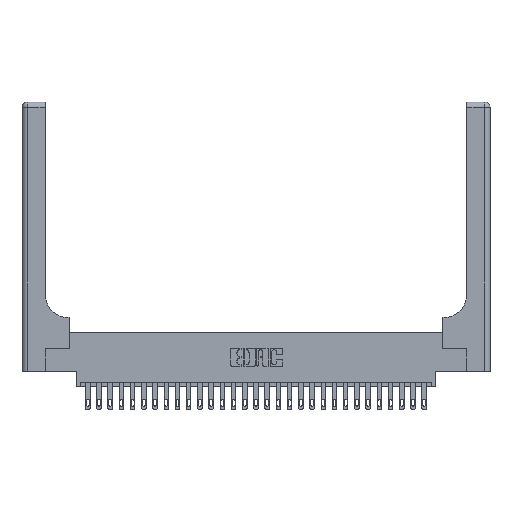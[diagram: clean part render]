
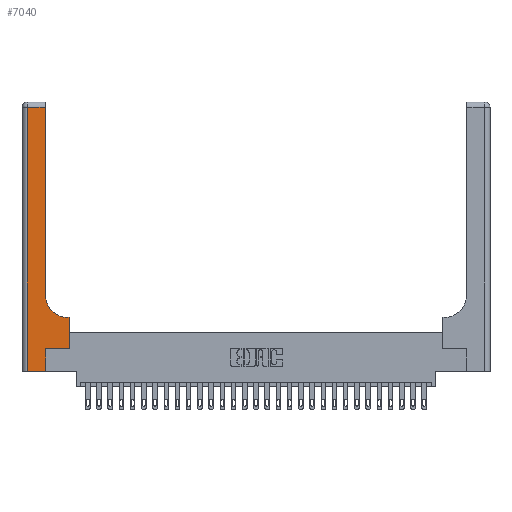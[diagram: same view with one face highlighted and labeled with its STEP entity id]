
A CAD part, top view. The second image highlights one B-rep face of the part: STEP entity #7040.
In plain terms, the highlighted planar face has unit normal (0, 0, 1).
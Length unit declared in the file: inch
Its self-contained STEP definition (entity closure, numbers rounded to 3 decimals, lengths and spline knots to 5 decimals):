
#105 = VERTEX_POINT ( 'NONE', #22768 ) ;
#300 = CARTESIAN_POINT ( 'NONE',  ( 0.528, 0.25, 0.37 ) ) ;
#528 = CARTESIAN_POINT ( 'NONE',  ( 0.265, 0., 0.37 ) ) ;
#1163 = EDGE_CURVE ( 'NONE', #9780, #12907, #8367, .T. ) ;
#1201 = ORIENTED_EDGE ( 'NONE', *, *, #1163, .T. ) ;
#1216 = DIRECTION ( 'NONE',  ( 1., 0., 0. ) ) ;
#1411 = LINE ( 'NONE', #24992, #21447 ) ;
#1665 = DIRECTION ( 'NONE',  ( 0., 0., -1. ) ) ;
#1756 = CARTESIAN_POINT ( 'NONE',  ( 0.26, 0.6, 0.37 ) ) ;
#2076 = PLANE ( 'NONE',  #18085 ) ;
#2388 = VECTOR ( 'NONE', #5751, 39.37008 ) ;
#2456 = VERTEX_POINT ( 'NONE', #13933 ) ;
#2569 = EDGE_CURVE ( 'NONE', #7289, #3537, #10303, .T. ) ;
#3537 = VERTEX_POINT ( 'NONE', #24204 ) ;
#3957 = EDGE_CURVE ( 'NONE', #3537, #9780, #1411, .T. ) ;
#4244 = ORIENTED_EDGE ( 'NONE', *, *, #14008, .T. ) ;
#5641 = CARTESIAN_POINT ( 'NONE',  ( 0.06, 0., 0.37 ) ) ;
#5751 = DIRECTION ( 'NONE',  ( 0., 1., 0. ) ) ;
#5802 = LINE ( 'NONE', #1756, #19402 ) ;
#6076 = DIRECTION ( 'NONE',  ( -1., 0., 0. ) ) ;
#6477 = ORIENTED_EDGE ( 'NONE', *, *, #21721, .T. ) ;
#6672 = EDGE_CURVE ( 'NONE', #21375, #105, #8628, .T. ) ;
#7040 = ADVANCED_FACE ( 'NONE', ( #18881 ), #2076, .F. ) ;
#7289 = VERTEX_POINT ( 'NONE', #15524 ) ;
#7384 = EDGE_CURVE ( 'NONE', #105, #17592, #5802, .T. ) ;
#7466 = DIRECTION ( 'NONE',  ( 0., 0., -1. ) ) ;
#7798 = VECTOR ( 'NONE', #10230, 39.37008 ) ;
#8081 = CARTESIAN_POINT ( 'NONE',  ( 0.26, 3., 0.37 ) ) ;
#8367 = LINE ( 'NONE', #16829, #20045 ) ;
#8628 = LINE ( 'NONE', #300, #20742 ) ;
#9693 = CARTESIAN_POINT ( 'NONE',  ( 0.51, 0.85, 0.37 ) ) ;
#9780 = VERTEX_POINT ( 'NONE', #13255 ) ;
#10230 = DIRECTION ( 'NONE',  ( 1., 0., 0. ) ) ;
#10303 = LINE ( 'NONE', #8081, #2388 ) ;
#11034 = EDGE_CURVE ( 'NONE', #12907, #12129, #13681, .T. ) ;
#11123 = DIRECTION ( 'NONE',  ( 0., 1., 0. ) ) ;
#11565 = CARTESIAN_POINT ( 'NONE',  ( 0.51, 0.6, 0.37 ) ) ;
#12129 = VERTEX_POINT ( 'NONE', #14837 ) ;
#12298 = EDGE_LOOP ( 'NONE', ( #26093, #23113, #1201, #16532, #6477, #4244, #24135, #21809, #20225 ) ) ;
#12312 = LINE ( 'NONE', #20792, #7798 ) ;
#12728 = AXIS2_PLACEMENT_3D ( 'NONE', #9693, #7466, #1216 ) ;
#12907 = VERTEX_POINT ( 'NONE', #5641 ) ;
#13255 = CARTESIAN_POINT ( 'NONE',  ( 0.06, 2.94, 0.37 ) ) ;
#13623 = CIRCLE ( 'NONE', #12728, 0.25 ) ;
#13681 = LINE ( 'NONE', #24087, #17603 ) ;
#13933 = CARTESIAN_POINT ( 'NONE',  ( 0.265, 0.25, 0.37 ) ) ;
#14008 = EDGE_CURVE ( 'NONE', #2456, #21375, #12312, .T. ) ;
#14052 = DIRECTION ( 'NONE',  ( -1., 0., 0. ) ) ;
#14837 = CARTESIAN_POINT ( 'NONE',  ( 0.265, 0., 0.37 ) ) ;
#15524 = CARTESIAN_POINT ( 'NONE',  ( 0.26, 0.85, 0.37 ) ) ;
#16505 = CARTESIAN_POINT ( 'NONE',  ( 0., 3., 0.37 ) ) ;
#16532 = ORIENTED_EDGE ( 'NONE', *, *, #11034, .T. ) ;
#16674 = LINE ( 'NONE', #528, #21599 ) ;
#16829 = CARTESIAN_POINT ( 'NONE',  ( 0.06, 3., 0.37 ) ) ;
#16845 = CARTESIAN_POINT ( 'NONE',  ( 0.528, 0.25, 0.37 ) ) ;
#17592 = VERTEX_POINT ( 'NONE', #11565 ) ;
#17603 = VECTOR ( 'NONE', #22157, 39.37008 ) ;
#18085 = AXIS2_PLACEMENT_3D ( 'NONE', #16505, #1665, #18336 ) ;
#18336 = DIRECTION ( 'NONE',  ( -1., 0., 0. ) ) ;
#18881 = FACE_OUTER_BOUND ( 'NONE', #12298, .T. ) ;
#19402 = VECTOR ( 'NONE', #6076, 39.37008 ) ;
#20045 = VECTOR ( 'NONE', #25283, 39.37008 ) ;
#20225 = ORIENTED_EDGE ( 'NONE', *, *, #21791, .T. ) ;
#20742 = VECTOR ( 'NONE', #11123, 39.37008 ) ;
#20792 = CARTESIAN_POINT ( 'NONE',  ( 0.265, 0.25, 0.37 ) ) ;
#21375 = VERTEX_POINT ( 'NONE', #16845 ) ;
#21447 = VECTOR ( 'NONE', #14052, 39.37008 ) ;
#21599 = VECTOR ( 'NONE', #23985, 39.37008 ) ;
#21721 = EDGE_CURVE ( 'NONE', #12129, #2456, #16674, .T. ) ;
#21791 = EDGE_CURVE ( 'NONE', #17592, #7289, #13623, .T. ) ;
#21809 = ORIENTED_EDGE ( 'NONE', *, *, #7384, .T. ) ;
#22157 = DIRECTION ( 'NONE',  ( 1., 0., 0. ) ) ;
#22768 = CARTESIAN_POINT ( 'NONE',  ( 0.528, 0.6, 0.37 ) ) ;
#23113 = ORIENTED_EDGE ( 'NONE', *, *, #3957, .T. ) ;
#23985 = DIRECTION ( 'NONE',  ( 0., 1., 0. ) ) ;
#24087 = CARTESIAN_POINT ( 'NONE',  ( 0., 0., 0.37 ) ) ;
#24135 = ORIENTED_EDGE ( 'NONE', *, *, #6672, .T. ) ;
#24204 = CARTESIAN_POINT ( 'NONE',  ( 0.26, 2.94, 0.37 ) ) ;
#24992 = CARTESIAN_POINT ( 'NONE',  ( 0., 2.94, 0.37 ) ) ;
#25283 = DIRECTION ( 'NONE',  ( 0., -1., 0. ) ) ;
#26093 = ORIENTED_EDGE ( 'NONE', *, *, #2569, .T. ) ;
